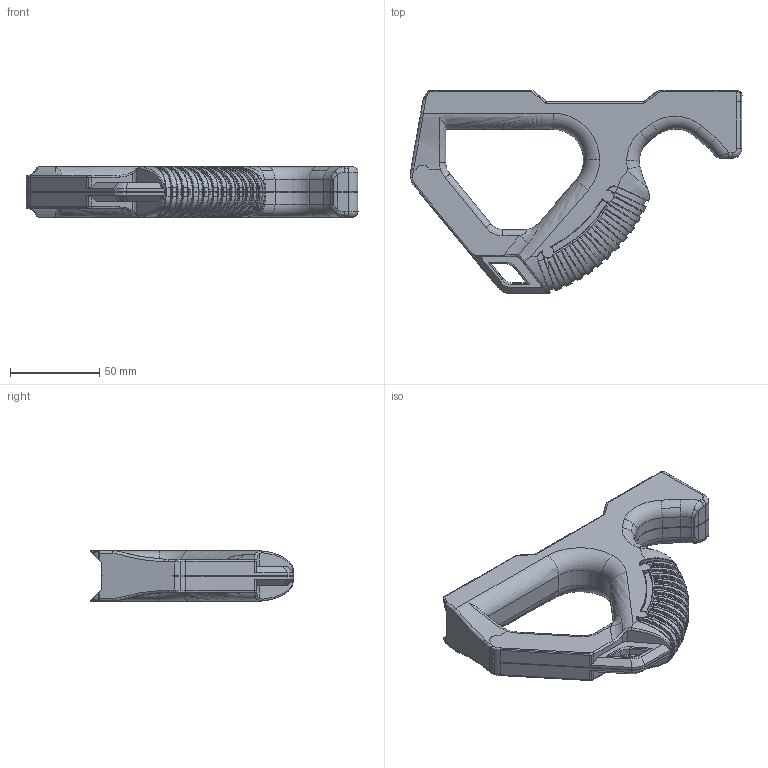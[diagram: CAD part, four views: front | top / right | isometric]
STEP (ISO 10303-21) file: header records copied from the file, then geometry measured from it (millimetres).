
FILE_DESCRIPTION (( 'STEP AP214' ), '1' );
FILE_NAME ('hera_cqr_.step', '2019-12-18T03:08:03', ( '' ), ( '' ), 'SwSTEP 2.0', 'SolidWorks 2019', '' );
FILE_SCHEMA (( 'AUTOMOTIVE_DESIGN' ));
Length unit declared in the file: millimetre
Products named in the file (1): hera_cqr_
Bounding box: 186 x 113.76 x 28.22 mm (x, y, z)
Volume: 221252.2 mm3; surface area: 38791.4 mm2
Topology: 1 solids, 1 shells, 1106 faces, 2728 edges, 1621 vertices
Faces by surface type: cylinder 371, cone 250, bspline 250, plane 196, torus 39
Entity records: 267833 total; most frequent: CARTESIAN_POINT 244633, ORIENTED_EDGE 5450, DIRECTION 3880, EDGE_CURVE 2725, VERTEX_POINT 1622, AXIS2_PLACEMENT_3D 1415, EDGE_LOOP 1111, ADVANCED_FACE 1106
